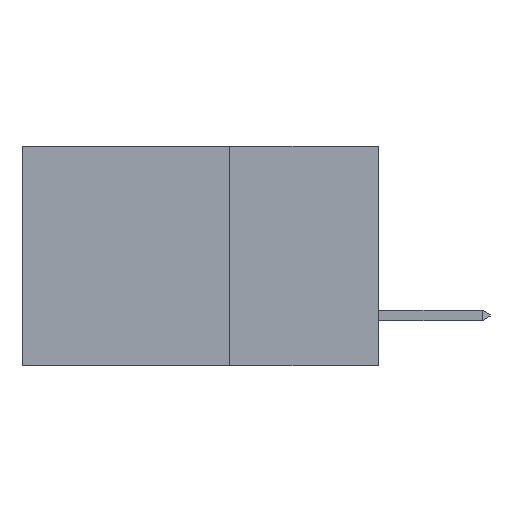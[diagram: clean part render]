
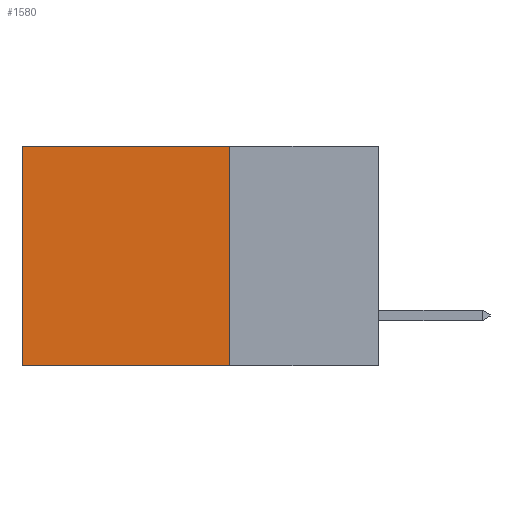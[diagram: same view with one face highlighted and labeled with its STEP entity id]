
A CAD part, left-side view. The second image highlights one B-rep face of the part: STEP entity #1580.
In plain terms, the highlighted planar face has unit normal (-1, 0, 0).
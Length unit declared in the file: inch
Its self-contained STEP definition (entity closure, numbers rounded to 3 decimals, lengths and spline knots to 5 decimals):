
#617 = DIRECTION ( 'NONE',  ( 0., 0., -1. ) ) ;
#660 = AXIS2_PLACEMENT_3D ( 'NONE', #20780, #20774, #20647 ) ;
#1353 = LINE ( 'NONE', #24654, #6166 ) ;
#1443 = EDGE_CURVE ( 'NONE', #10201, #5382, #22120, .T. ) ;
#1580 = ADVANCED_FACE ( 'NONE', ( #23682 ), #21749, .F. ) ;
#1726 = CARTESIAN_POINT ( 'NONE',  ( 0.298, 0.6, 0. ) ) ;
#4051 = ORIENTED_EDGE ( 'NONE', *, *, #1443, .F. ) ;
#5382 = VERTEX_POINT ( 'NONE', #13030 ) ;
#6166 = VECTOR ( 'NONE', #8372, 39.37008 ) ;
#6422 = ORIENTED_EDGE ( 'NONE', *, *, #20638, .F. ) ;
#8372 = DIRECTION ( 'NONE',  ( 0., 0., -1. ) ) ;
#8719 = EDGE_CURVE ( 'NONE', #10201, #24957, #9155, .T. ) ;
#9155 = LINE ( 'NONE', #23617, #19405 ) ;
#9367 = CARTESIAN_POINT ( 'NONE',  ( 0.298, 0.25, 0. ) ) ;
#10201 = VERTEX_POINT ( 'NONE', #20057 ) ;
#12014 = CARTESIAN_POINT ( 'NONE',  ( 0.298, 0.6, -0.37 ) ) ;
#12677 = VECTOR ( 'NONE', #16673, 39.37008 ) ;
#13030 = CARTESIAN_POINT ( 'NONE',  ( 0.298, 0.25, -0.37 ) ) ;
#13289 = EDGE_LOOP ( 'NONE', ( #19944, #6422, #4051, #17298 ) ) ;
#13298 = LINE ( 'NONE', #14567, #12677 ) ;
#14567 = CARTESIAN_POINT ( 'NONE',  ( 0.298, 0.25, -0.37 ) ) ;
#16673 = DIRECTION ( 'NONE',  ( 0., 1., 0. ) ) ;
#16740 = VECTOR ( 'NONE', #617, 39.37008 ) ;
#17069 = EDGE_CURVE ( 'NONE', #24957, #21779, #1353, .T. ) ;
#17298 = ORIENTED_EDGE ( 'NONE', *, *, #8719, .T. ) ;
#19405 = VECTOR ( 'NONE', #25628, 39.37008 ) ;
#19944 = ORIENTED_EDGE ( 'NONE', *, *, #17069, .T. ) ;
#20057 = CARTESIAN_POINT ( 'NONE',  ( 0.298, 0.25, 0. ) ) ;
#20638 = EDGE_CURVE ( 'NONE', #5382, #21779, #13298, .T. ) ;
#20647 = DIRECTION ( 'NONE',  ( 0., 0., -1. ) ) ;
#20774 = DIRECTION ( 'NONE',  ( 1., 0., 0. ) ) ;
#20780 = CARTESIAN_POINT ( 'NONE',  ( 0.298, 0.25, 0. ) ) ;
#21749 = PLANE ( 'NONE',  #660 ) ;
#21779 = VERTEX_POINT ( 'NONE', #12014 ) ;
#22120 = LINE ( 'NONE', #9367, #16740 ) ;
#23617 = CARTESIAN_POINT ( 'NONE',  ( 0.298, 0.25, 0. ) ) ;
#23682 = FACE_OUTER_BOUND ( 'NONE', #13289, .T. ) ;
#24654 = CARTESIAN_POINT ( 'NONE',  ( 0.298, 0.6, 0. ) ) ;
#24957 = VERTEX_POINT ( 'NONE', #1726 ) ;
#25628 = DIRECTION ( 'NONE',  ( 0., 1., 0. ) ) ;
